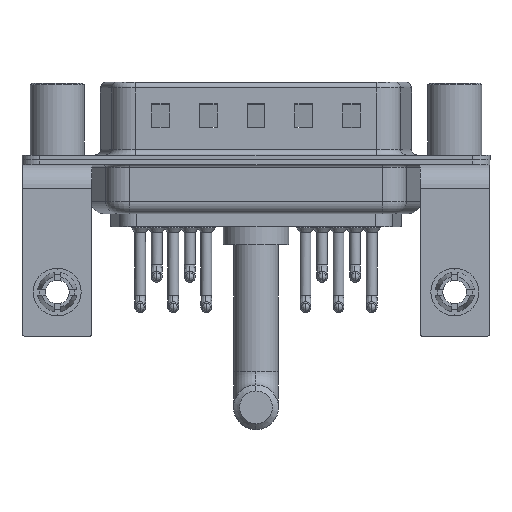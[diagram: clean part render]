
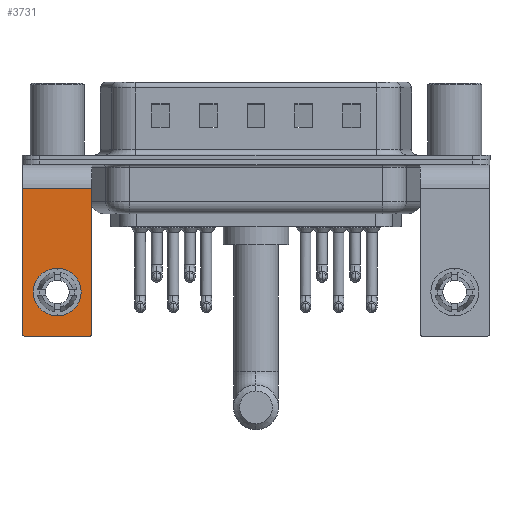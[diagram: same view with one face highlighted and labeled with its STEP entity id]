
A CAD part, front view. The second image highlights one B-rep face of the part: STEP entity #3731.
In plain terms, the highlighted planar face has unit normal (0, -1, 0).
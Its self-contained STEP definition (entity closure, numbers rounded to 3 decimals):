
#17 = VERTEX_POINT ( 'NONE', #18838 ) ;
#660 = EDGE_LOOP ( 'NONE', ( #21236, #7334 ) ) ;
#1618 = DIRECTION ( 'NONE',  ( 0., -1., 0. ) ) ;
#1647 = LINE ( 'NONE', #13599, #11769 ) ;
#2292 = DIRECTION ( 'NONE',  ( 0., 1., 0. ) ) ;
#2676 = CARTESIAN_POINT ( 'NONE',  ( 0., -6.25, -11.07 ) ) ;
#2803 = LINE ( 'NONE', #23400, #4223 ) ;
#3015 = AXIS2_PLACEMENT_3D ( 'NONE', #7626, #3680, #25836 ) ;
#3209 = EDGE_CURVE ( 'NONE', #14040, #17, #2803, .T. ) ;
#3331 = EDGE_CURVE ( 'NONE', #14040, #16138, #13902, .T. ) ;
#3426 = FACE_BOUND ( 'NONE', #660, .T. ) ;
#3557 = ORIENTED_EDGE ( 'NONE', *, *, #10436, .T. ) ;
#3680 = DIRECTION ( 'NONE',  ( 0., 1., 0. ) ) ;
#3731 = ADVANCED_FACE ( 'NONE', ( #3426, #5648 ), #5778, .F. ) ;
#3861 = CARTESIAN_POINT ( 'NONE',  ( 0., -6.25, -13.07 ) ) ;
#4097 = CIRCLE ( 'NONE', #12060, 2. ) ;
#4223 = VECTOR ( 'NONE', #16840, 1000. ) ;
#4247 = ORIENTED_EDGE ( 'NONE', *, *, #8532, .T. ) ;
#4930 = VECTOR ( 'NONE', #17478, 1000. ) ;
#5419 = CARTESIAN_POINT ( 'NONE',  ( -2.9, -6.25, -2.4 ) ) ;
#5648 = FACE_OUTER_BOUND ( 'NONE', #11507, .T. ) ;
#5778 = PLANE ( 'NONE',  #3015 ) ;
#7334 = ORIENTED_EDGE ( 'NONE', *, *, #10334, .T. ) ;
#7409 = ORIENTED_EDGE ( 'NONE', *, *, #11365, .T. ) ;
#7626 = CARTESIAN_POINT ( 'NONE',  ( 2.9, -6.25, -2.4 ) ) ;
#8026 = VERTEX_POINT ( 'NONE', #3861 ) ;
#8329 = CARTESIAN_POINT ( 'NONE',  ( -2.65, -6.25, -14.55 ) ) ;
#8532 = EDGE_CURVE ( 'NONE', #22535, #11960, #17611, .T. ) ;
#8938 = CARTESIAN_POINT ( 'NONE',  ( 2.9, -6.25, -14.55 ) ) ;
#9302 = CIRCLE ( 'NONE', #23979, 2. ) ;
#10334 = EDGE_CURVE ( 'NONE', #13676, #8026, #9302, .T. ) ;
#10436 = EDGE_CURVE ( 'NONE', #11960, #17, #15207, .T. ) ;
#11270 = CARTESIAN_POINT ( 'NONE',  ( 2.9, -6.25, -2.4 ) ) ;
#11365 = EDGE_CURVE ( 'NONE', #19960, #22535, #1647, .T. ) ;
#11480 = DIRECTION ( 'NONE',  ( -1., 0., 0. ) ) ;
#11507 = EDGE_LOOP ( 'NONE', ( #4247, #3557, #23948, #18277, #21438, #7409 ) ) ;
#11769 = VECTOR ( 'NONE', #11480, 1000. ) ;
#11960 = VERTEX_POINT ( 'NONE', #23914 ) ;
#12060 = AXIS2_PLACEMENT_3D ( 'NONE', #19887, #18168, #23690 ) ;
#13599 = CARTESIAN_POINT ( 'NONE',  ( 2.9, -6.25, -2.4 ) ) ;
#13676 = VERTEX_POINT ( 'NONE', #23114 ) ;
#13902 = CIRCLE ( 'NONE', #14319, 0.25 ) ;
#14040 = VERTEX_POINT ( 'NONE', #20739 ) ;
#14319 = AXIS2_PLACEMENT_3D ( 'NONE', #19850, #1618, #17615 ) ;
#14368 = DIRECTION ( 'NONE',  ( 0., 0., 1. ) ) ;
#14877 = VECTOR ( 'NONE', #25259, 1000. ) ;
#15207 = CIRCLE ( 'NONE', #25243, 0.25 ) ;
#16138 = VERTEX_POINT ( 'NONE', #8938 ) ;
#16332 = DIRECTION ( 'NONE',  ( 0., -1., 0. ) ) ;
#16840 = DIRECTION ( 'NONE',  ( -1., 0., 0. ) ) ;
#17132 = CARTESIAN_POINT ( 'NONE',  ( 2.9, -6.25, -2.4 ) ) ;
#17478 = DIRECTION ( 'NONE',  ( 0., 0., -1. ) ) ;
#17496 = EDGE_CURVE ( 'NONE', #19960, #16138, #19089, .T. ) ;
#17611 = LINE ( 'NONE', #5419, #4930 ) ;
#17615 = DIRECTION ( 'NONE',  ( 0., 0., 1. ) ) ;
#18168 = DIRECTION ( 'NONE',  ( 0., 1., 0. ) ) ;
#18277 = ORIENTED_EDGE ( 'NONE', *, *, #3331, .T. ) ;
#18838 = CARTESIAN_POINT ( 'NONE',  ( -2.65, -6.25, -14.8 ) ) ;
#18928 = DIRECTION ( 'NONE',  ( 0., 0., 1. ) ) ;
#19089 = LINE ( 'NONE', #17132, #14877 ) ;
#19850 = CARTESIAN_POINT ( 'NONE',  ( 2.65, -6.25, -14.55 ) ) ;
#19887 = CARTESIAN_POINT ( 'NONE',  ( 0., -6.25, -11.07 ) ) ;
#19960 = VERTEX_POINT ( 'NONE', #11270 ) ;
#20547 = EDGE_CURVE ( 'NONE', #8026, #13676, #4097, .T. ) ;
#20739 = CARTESIAN_POINT ( 'NONE',  ( 2.65, -6.25, -14.8 ) ) ;
#21236 = ORIENTED_EDGE ( 'NONE', *, *, #20547, .T. ) ;
#21438 = ORIENTED_EDGE ( 'NONE', *, *, #17496, .F. ) ;
#22535 = VERTEX_POINT ( 'NONE', #23147 ) ;
#23114 = CARTESIAN_POINT ( 'NONE',  ( 0., -6.25, -9.07 ) ) ;
#23147 = CARTESIAN_POINT ( 'NONE',  ( -2.9, -6.25, -2.4 ) ) ;
#23400 = CARTESIAN_POINT ( 'NONE',  ( 2.9, -6.25, -14.8 ) ) ;
#23690 = DIRECTION ( 'NONE',  ( 0., 0., 1. ) ) ;
#23914 = CARTESIAN_POINT ( 'NONE',  ( -2.9, -6.25, -14.55 ) ) ;
#23948 = ORIENTED_EDGE ( 'NONE', *, *, #3209, .F. ) ;
#23979 = AXIS2_PLACEMENT_3D ( 'NONE', #2676, #2292, #14368 ) ;
#25243 = AXIS2_PLACEMENT_3D ( 'NONE', #8329, #16332, #18928 ) ;
#25259 = DIRECTION ( 'NONE',  ( 0., 0., -1. ) ) ;
#25836 = DIRECTION ( 'NONE',  ( 0., 0., 1. ) ) ;
